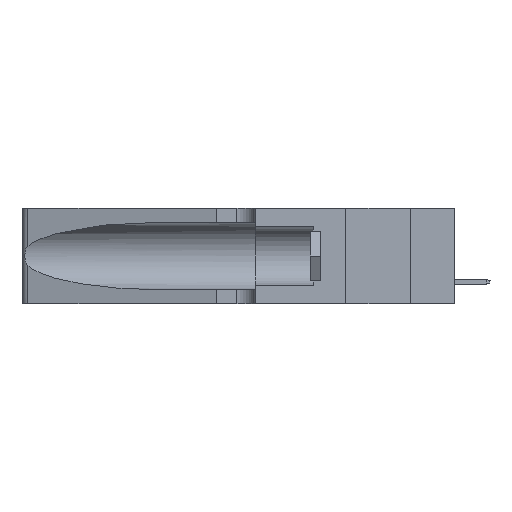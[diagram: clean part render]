
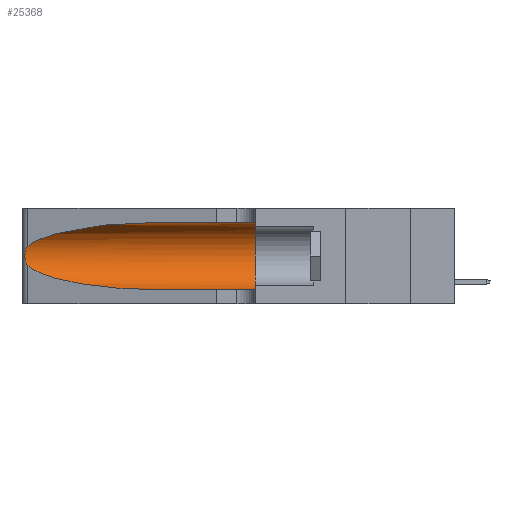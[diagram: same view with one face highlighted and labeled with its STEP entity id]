
A CAD part, left-side view. The second image highlights one B-rep face of the part: STEP entity #25368.
In plain terms, the highlighted cylindrical face has radius 3.308 mm (diameter 6.617 mm), a partial arc.
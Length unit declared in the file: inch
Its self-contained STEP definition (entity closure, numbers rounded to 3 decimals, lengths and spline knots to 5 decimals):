
#869 = ORIENTED_EDGE ( 'NONE', *, *, #9612, .T. ) ;
#1166 = DIRECTION ( 'NONE',  ( 0., -1., 0. ) ) ;
#1456 = EDGE_CURVE ( 'NONE', #7826, #4421, #3991, .T. ) ;
#1996 = ORIENTED_EDGE ( 'NONE', *, *, #8220, .T. ) ;
#2251 = CARTESIAN_POINT ( 'NONE',  ( 0.2373, 1.15595, 0.08982 ) ) ;
#3563 = CARTESIAN_POINT ( 'NONE',  ( 0.25487, 1.22718, 0.22369 ) ) ;
#3773 = EDGE_CURVE ( 'NONE', #32040, #31015, #13880, .T. ) ;
#3991 =( BOUNDED_CURVE ( )  B_SPLINE_CURVE ( 3, ( #6263, #2251, #27478, #11751 ),
 .UNSPECIFIED., .F., .F. ) 
 B_SPLINE_CURVE_WITH_KNOTS ( ( 4, 4 ),
 ( 3.44316, 4.71239 ),
 .UNSPECIFIED. ) 
 CURVE ( )  GEOMETRIC_REPRESENTATION_ITEM ( )  RATIONAL_B_SPLINE_CURVE ( ( 1., 0.87, 0.87, 1. ) ) 
 REPRESENTATION_ITEM ( '' )  );
#4421 = VERTEX_POINT ( 'NONE', #7872 ) ;
#5616 = ORIENTED_EDGE ( 'NONE', *, *, #14333, .T. ) ;
#6056 = CARTESIAN_POINT ( 'NONE',  ( 0.18966, 0.96281, 0.31525 ) ) ;
#6263 = CARTESIAN_POINT ( 'NONE',  ( 0.25487, 1.22718, 0.14631 ) ) ;
#6819 = CYLINDRICAL_SURFACE ( 'NONE', #8861, 0.13025 ) ;
#7618 = CARTESIAN_POINT ( 'NONE',  ( 0.1305, 0.35, 0.31525 ) ) ;
#7826 = VERTEX_POINT ( 'NONE', #26333 ) ;
#7872 = CARTESIAN_POINT ( 'NONE',  ( 0.1305, 0.72297, 0.05475 ) ) ;
#8129 = LINE ( 'NONE', #22872, #11971 ) ;
#8220 = EDGE_CURVE ( 'NONE', #4421, #22079, #8129, .T. ) ;
#8621 = CARTESIAN_POINT ( 'NONE',  ( 0.25487, 1.22718, 0.14631 ) ) ;
#8783 = CARTESIAN_POINT ( 'NONE',  ( 0.25639, 1.23184, 0.21858 ) ) ;
#8861 = AXIS2_PLACEMENT_3D ( 'NONE', #9133, #1166, #21401 ) ;
#9133 = CARTESIAN_POINT ( 'NONE',  ( 0.1305, 1.61858, 0.185 ) ) ;
#9167 = VERTEX_POINT ( 'NONE', #11989 ) ;
#9408 = CARTESIAN_POINT ( 'NONE',  ( 0.25487, 1.22718, 0.22369 ) ) ;
#9612 = EDGE_CURVE ( 'NONE', #9167, #7826, #23798, .T. ) ;
#9904 =( BOUNDED_CURVE ( )  B_SPLINE_CURVE ( 3, ( #25805, #6056, #13373, #3563 ),
 .UNSPECIFIED., .F., .T. ) 
 B_SPLINE_CURVE_WITH_KNOTS ( ( 4, 4 ),
 ( 1.5708, 2.84003 ),
 .UNSPECIFIED. ) 
 CURVE ( )  GEOMETRIC_REPRESENTATION_ITEM ( )  RATIONAL_B_SPLINE_CURVE ( ( 1., 0.87, 0.87, 1. ) ) 
 REPRESENTATION_ITEM ( '' )  );
#10130 = DIRECTION ( 'NONE',  ( 0., -1., 0. ) ) ;
#10973 = CARTESIAN_POINT ( 'NONE',  ( 0.26017, 1.23833, 0.17102 ) ) ;
#11751 = CARTESIAN_POINT ( 'NONE',  ( 0.1305, 0.72297, 0.05475 ) ) ;
#11971 = VECTOR ( 'NONE', #10130, 39.37008 ) ;
#11989 = CARTESIAN_POINT ( 'NONE',  ( 0.25487, 1.22718, 0.22369 ) ) ;
#13373 = CARTESIAN_POINT ( 'NONE',  ( 0.2373, 1.15595, 0.28018 ) ) ;
#13880 = LINE ( 'NONE', #16850, #26116 ) ;
#14333 = EDGE_CURVE ( 'NONE', #32040, #9167, #9904, .T. ) ;
#15536 = CIRCLE ( 'NONE', #21866, 0.13025 ) ;
#15959 = EDGE_LOOP ( 'NONE', ( #5616, #869, #26518, #1996, #31184, #17686 ) ) ;
#16850 = CARTESIAN_POINT ( 'NONE',  ( 0.1305, 1.61858, 0.31525 ) ) ;
#17686 = ORIENTED_EDGE ( 'NONE', *, *, #3773, .F. ) ;
#18769 = FACE_OUTER_BOUND ( 'NONE', #15959, .T. ) ;
#18878 = EDGE_CURVE ( 'NONE', #31015, #22079, #15536, .T. ) ;
#18907 = CARTESIAN_POINT ( 'NONE',  ( 0.26075, 1.23896, 0.19203 ) ) ;
#18960 = DIRECTION ( 'NONE',  ( 0., 0., 1. ) ) ;
#21070 = CARTESIAN_POINT ( 'NONE',  ( 0.25856, 1.23593, 0.16098 ) ) ;
#21220 = CARTESIAN_POINT ( 'NONE',  ( 0.26075, 1.23896, 0.178 ) ) ;
#21379 = CARTESIAN_POINT ( 'NONE',  ( 0.25854, 1.2359, 0.20912 ) ) ;
#21401 = DIRECTION ( 'NONE',  ( 0., 0., -1. ) ) ;
#21445 = CARTESIAN_POINT ( 'NONE',  ( 0.1305, 0.35, 0.185 ) ) ;
#21866 = AXIS2_PLACEMENT_3D ( 'NONE', #21445, #26748, #18960 ) ;
#22079 = VERTEX_POINT ( 'NONE', #30676 ) ;
#22872 = CARTESIAN_POINT ( 'NONE',  ( 0.1305, 1.61858, 0.05475 ) ) ;
#23798 = B_SPLINE_CURVE_WITH_KNOTS ( 'NONE', 3,
 ( #9408, #31482, #8783, #28856, #21379, #31003, #18907, #21220, #10973, #21070, #31315, #29023, #31158, #8621 ),
 .UNSPECIFIED., .F., .F.,
 ( 4, 2, 2, 2, 2, 2, 4 ),
 ( 0., 0.00027, 0.00053, 0.00107, 0.0016, 0.00187, 0.00214 ),
 .UNSPECIFIED. ) ;
#25368 = ADVANCED_FACE ( 'NONE', ( #18769 ), #6819, .F. ) ;
#25805 = CARTESIAN_POINT ( 'NONE',  ( 0.1305, 0.72297, 0.31525 ) ) ;
#26116 = VECTOR ( 'NONE', #29589, 39.37008 ) ;
#26333 = CARTESIAN_POINT ( 'NONE',  ( 0.25487, 1.22718, 0.14631 ) ) ;
#26518 = ORIENTED_EDGE ( 'NONE', *, *, #1456, .T. ) ;
#26748 = DIRECTION ( 'NONE',  ( 0., 1., 0. ) ) ;
#27478 = CARTESIAN_POINT ( 'NONE',  ( 0.18966, 0.96281, 0.05475 ) ) ;
#28721 = CARTESIAN_POINT ( 'NONE',  ( 0.1305, 0.72297, 0.31525 ) ) ;
#28856 = CARTESIAN_POINT ( 'NONE',  ( 0.25787, 1.23484, 0.2124 ) ) ;
#29023 = CARTESIAN_POINT ( 'NONE',  ( 0.25639, 1.23186, 0.15144 ) ) ;
#29589 = DIRECTION ( 'NONE',  ( 0., -1., 0. ) ) ;
#30676 = CARTESIAN_POINT ( 'NONE',  ( 0.1305, 0.35, 0.05475 ) ) ;
#31003 = CARTESIAN_POINT ( 'NONE',  ( 0.26018, 1.23835, 0.19895 ) ) ;
#31015 = VERTEX_POINT ( 'NONE', #7618 ) ;
#31158 = CARTESIAN_POINT ( 'NONE',  ( 0.25555, 1.22993, 0.14849 ) ) ;
#31184 = ORIENTED_EDGE ( 'NONE', *, *, #18878, .F. ) ;
#31315 = CARTESIAN_POINT ( 'NONE',  ( 0.25789, 1.23486, 0.15765 ) ) ;
#31482 = CARTESIAN_POINT ( 'NONE',  ( 0.25555, 1.22994, 0.2215 ) ) ;
#32040 = VERTEX_POINT ( 'NONE', #28721 ) ;
